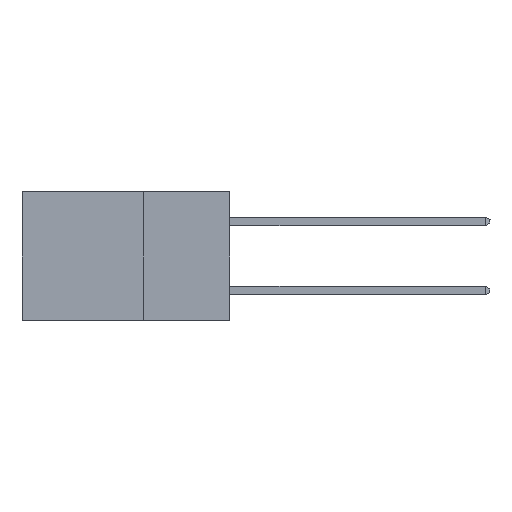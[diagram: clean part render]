
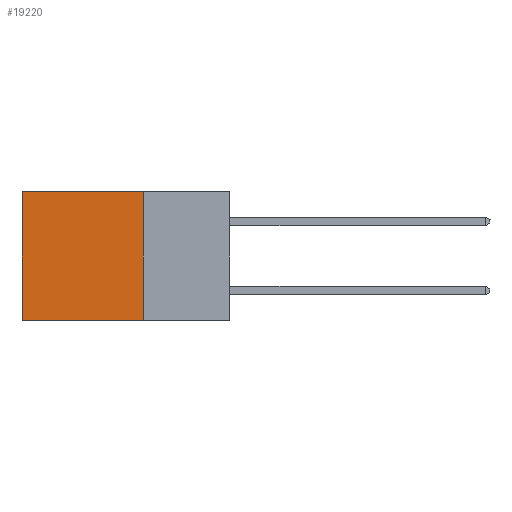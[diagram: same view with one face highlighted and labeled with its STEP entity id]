
A CAD part, left-side view. The second image highlights one B-rep face of the part: STEP entity #19220.
In plain terms, the highlighted planar face has unit normal (-1, 0, 0).
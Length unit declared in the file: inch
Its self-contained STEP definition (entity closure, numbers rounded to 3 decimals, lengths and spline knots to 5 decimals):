
#486 = AXIS2_PLACEMENT_3D ( 'NONE', #4585, #15756, #4778 ) ;
#965 = DIRECTION ( 'NONE',  ( 0., 0., -1. ) ) ;
#1034 = VECTOR ( 'NONE', #8615, 39.37008 ) ;
#1906 = CARTESIAN_POINT ( 'NONE',  ( 0.2615, 0.25, 0. ) ) ;
#2557 = VECTOR ( 'NONE', #14703, 39.37008 ) ;
#2642 = CARTESIAN_POINT ( 'NONE',  ( 0.2615, 0.25, -0.37 ) ) ;
#3712 = VERTEX_POINT ( 'NONE', #20669 ) ;
#4530 = ORIENTED_EDGE ( 'NONE', *, *, #6467, .F. ) ;
#4585 = CARTESIAN_POINT ( 'NONE',  ( 0.2615, 0.25, -0.37 ) ) ;
#4778 = DIRECTION ( 'NONE',  ( 0., 0., -1. ) ) ;
#4879 = CARTESIAN_POINT ( 'NONE',  ( 0.2615, 0.25, -0.37 ) ) ;
#5813 = VERTEX_POINT ( 'NONE', #12065 ) ;
#6467 = EDGE_CURVE ( 'NONE', #18495, #5813, #10654, .T. ) ;
#8163 = CARTESIAN_POINT ( 'NONE',  ( 0.2615, 0.25, 0. ) ) ;
#8438 = ORIENTED_EDGE ( 'NONE', *, *, #19346, .F. ) ;
#8550 = ORIENTED_EDGE ( 'NONE', *, *, #11206, .T. ) ;
#8615 = DIRECTION ( 'NONE',  ( 0., 0., -1. ) ) ;
#9712 = CARTESIAN_POINT ( 'NONE',  ( 0.2615, 0.6, 0. ) ) ;
#10654 = LINE ( 'NONE', #2642, #16837 ) ;
#11206 = EDGE_CURVE ( 'NONE', #18495, #18519, #11429, .T. ) ;
#11416 = LINE ( 'NONE', #4879, #2557 ) ;
#11429 = LINE ( 'NONE', #8163, #17544 ) ;
#11647 = DIRECTION ( 'NONE',  ( 0., 1., 0. ) ) ;
#11761 = CARTESIAN_POINT ( 'NONE',  ( 0.2615, 0.6, -0.37 ) ) ;
#11874 = ORIENTED_EDGE ( 'NONE', *, *, #12708, .T. ) ;
#12065 = CARTESIAN_POINT ( 'NONE',  ( 0.2615, 0.25, -0.37 ) ) ;
#12708 = EDGE_CURVE ( 'NONE', #18519, #3712, #19913, .T. ) ;
#13921 = EDGE_LOOP ( 'NONE', ( #11874, #8438, #4530, #8550 ) ) ;
#14082 = PLANE ( 'NONE',  #486 ) ;
#14703 = DIRECTION ( 'NONE',  ( 0., 1., 0. ) ) ;
#15756 = DIRECTION ( 'NONE',  ( 1., 0., 0. ) ) ;
#16837 = VECTOR ( 'NONE', #965, 39.37008 ) ;
#17544 = VECTOR ( 'NONE', #11647, 39.37008 ) ;
#18495 = VERTEX_POINT ( 'NONE', #1906 ) ;
#18519 = VERTEX_POINT ( 'NONE', #9712 ) ;
#19036 = FACE_OUTER_BOUND ( 'NONE', #13921, .T. ) ;
#19220 = ADVANCED_FACE ( 'NONE', ( #19036 ), #14082, .F. ) ;
#19346 = EDGE_CURVE ( 'NONE', #5813, #3712, #11416, .T. ) ;
#19913 = LINE ( 'NONE', #11761, #1034 ) ;
#20669 = CARTESIAN_POINT ( 'NONE',  ( 0.2615, 0.6, -0.37 ) ) ;
